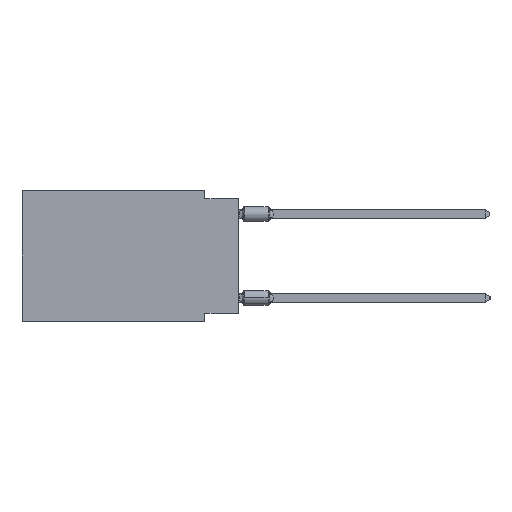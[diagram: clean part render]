
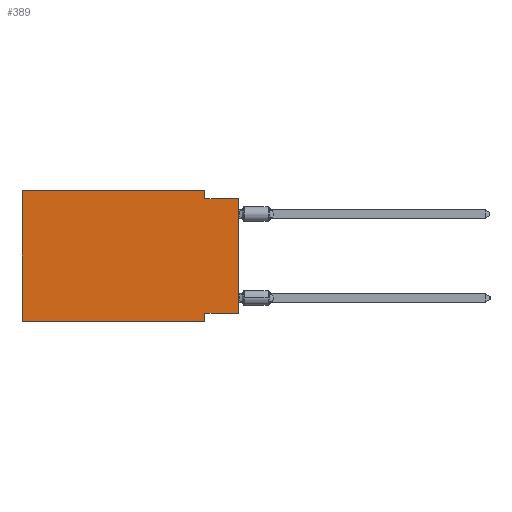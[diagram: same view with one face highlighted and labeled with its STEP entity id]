
A CAD part, left-side view. The second image highlights one B-rep face of the part: STEP entity #389.
In plain terms, the highlighted planar face has unit normal (-1, 0, 0).
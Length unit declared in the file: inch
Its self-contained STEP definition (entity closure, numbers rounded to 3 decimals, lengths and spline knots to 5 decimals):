
#389 = ADVANCED_FACE ( 'NONE', ( #33586 ), #12713, .F. ) ;
#676 = DIRECTION ( 'NONE',  ( 0., 0., -1. ) ) ;
#1525 = LINE ( 'NONE', #18346, #25292 ) ;
#1599 = ORIENTED_EDGE ( 'NONE', *, *, #51982, .F. ) ;
#2204 = LINE ( 'NONE', #40421, #5563 ) ;
#2867 = ORIENTED_EDGE ( 'NONE', *, *, #32821, .F. ) ;
#4203 = LINE ( 'NONE', #37288, #9433 ) ;
#4791 = DIRECTION ( 'NONE',  ( 0., -1., 0. ) ) ;
#5366 = VECTOR ( 'NONE', #4791, 39.37008 ) ;
#5379 = ORIENTED_EDGE ( 'NONE', *, *, #10379, .F. ) ;
#5563 = VECTOR ( 'NONE', #47493, 39.37008 ) ;
#5771 = VERTEX_POINT ( 'NONE', #19078 ) ;
#5772 = VERTEX_POINT ( 'NONE', #31256 ) ;
#6531 = EDGE_CURVE ( 'NONE', #24821, #45064, #47139, .T. ) ;
#7107 = EDGE_LOOP ( 'NONE', ( #31447, #1599, #49601, #21520, #13195, #26728, #2867, #5379 ) ) ;
#8909 = DIRECTION ( 'NONE',  ( 1., 0., 0. ) ) ;
#9433 = VECTOR ( 'NONE', #676, 39.37008 ) ;
#10106 = VERTEX_POINT ( 'NONE', #41285 ) ;
#10379 = EDGE_CURVE ( 'NONE', #24821, #10106, #2204, .T. ) ;
#11289 = CARTESIAN_POINT ( 'NONE',  ( 0., 0., -0.365 ) ) ;
#12713 = PLANE ( 'NONE',  #19572 ) ;
#13195 = ORIENTED_EDGE ( 'NONE', *, *, #27670, .F. ) ;
#14047 = CARTESIAN_POINT ( 'NONE',  ( 0., 0., 0. ) ) ;
#15847 = LINE ( 'NONE', #53291, #31678 ) ;
#18346 = CARTESIAN_POINT ( 'NONE',  ( 0., 0., -0.025 ) ) ;
#18827 = VECTOR ( 'NONE', #43872, 39.37008 ) ;
#19078 = CARTESIAN_POINT ( 'NONE',  ( 0., 0.1, 0. ) ) ;
#19572 = AXIS2_PLACEMENT_3D ( 'NONE', #46335, #8909, #33045 ) ;
#21520 = ORIENTED_EDGE ( 'NONE', *, *, #51943, .F. ) ;
#22708 = LINE ( 'NONE', #47107, #28695 ) ;
#23482 = DIRECTION ( 'NONE',  ( 0., 0., -1. ) ) ;
#23749 = CARTESIAN_POINT ( 'NONE',  ( 0., 0.1, 0. ) ) ;
#24821 = VERTEX_POINT ( 'NONE', #11289 ) ;
#25292 = VECTOR ( 'NONE', #43283, 39.37008 ) ;
#25676 = CARTESIAN_POINT ( 'NONE',  ( 0., 0.1, -0.39 ) ) ;
#26728 = ORIENTED_EDGE ( 'NONE', *, *, #51144, .T. ) ;
#27670 = EDGE_CURVE ( 'NONE', #5772, #29625, #15847, .T. ) ;
#28695 = VECTOR ( 'NONE', #34623, 39.37008 ) ;
#29280 = CARTESIAN_POINT ( 'NONE',  ( 0., 0., -0.025 ) ) ;
#29625 = VERTEX_POINT ( 'NONE', #33941 ) ;
#31256 = CARTESIAN_POINT ( 'NONE',  ( 0., 0.645, -0.39 ) ) ;
#31447 = ORIENTED_EDGE ( 'NONE', *, *, #6531, .T. ) ;
#31678 = VECTOR ( 'NONE', #40536, 39.37008 ) ;
#32821 = EDGE_CURVE ( 'NONE', #10106, #36873, #4203, .T. ) ;
#33045 = DIRECTION ( 'NONE',  ( 0., 0., -1. ) ) ;
#33586 = FACE_OUTER_BOUND ( 'NONE', #7107, .T. ) ;
#33941 = CARTESIAN_POINT ( 'NONE',  ( 0., 0.645, 0. ) ) ;
#34623 = DIRECTION ( 'NONE',  ( 0., -1., 0. ) ) ;
#35904 = VERTEX_POINT ( 'NONE', #36740 ) ;
#36740 = CARTESIAN_POINT ( 'NONE',  ( 0., 0.1, -0.025 ) ) ;
#36873 = VERTEX_POINT ( 'NONE', #25676 ) ;
#37070 = EDGE_CURVE ( 'NONE', #5771, #35904, #52528, .T. ) ;
#37288 = CARTESIAN_POINT ( 'NONE',  ( 0., 0.1, -0.39 ) ) ;
#40421 = CARTESIAN_POINT ( 'NONE',  ( 0., 0., -0.365 ) ) ;
#40536 = DIRECTION ( 'NONE',  ( 0., 0., 1. ) ) ;
#41285 = CARTESIAN_POINT ( 'NONE',  ( 0., 0.1, -0.365 ) ) ;
#41945 = CARTESIAN_POINT ( 'NONE',  ( 0., 0.645, 0. ) ) ;
#43283 = DIRECTION ( 'NONE',  ( 0., -1., 0. ) ) ;
#43872 = DIRECTION ( 'NONE',  ( 0., 0., 1. ) ) ;
#45064 = VERTEX_POINT ( 'NONE', #29280 ) ;
#46008 = LINE ( 'NONE', #41945, #5366 ) ;
#46335 = CARTESIAN_POINT ( 'NONE',  ( 0., 0.645, 0. ) ) ;
#47107 = CARTESIAN_POINT ( 'NONE',  ( 0., 0.645, -0.39 ) ) ;
#47139 = LINE ( 'NONE', #14047, #18827 ) ;
#47493 = DIRECTION ( 'NONE',  ( 0., 1., 0. ) ) ;
#48683 = VECTOR ( 'NONE', #23482, 39.37008 ) ;
#49601 = ORIENTED_EDGE ( 'NONE', *, *, #37070, .F. ) ;
#51144 = EDGE_CURVE ( 'NONE', #5772, #36873, #22708, .T. ) ;
#51943 = EDGE_CURVE ( 'NONE', #29625, #5771, #46008, .T. ) ;
#51982 = EDGE_CURVE ( 'NONE', #35904, #45064, #1525, .T. ) ;
#52528 = LINE ( 'NONE', #23749, #48683 ) ;
#53291 = CARTESIAN_POINT ( 'NONE',  ( 0., 0.645, 0. ) ) ;
